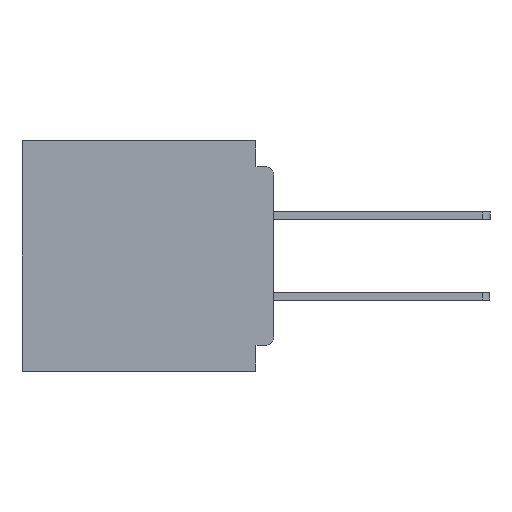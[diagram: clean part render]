
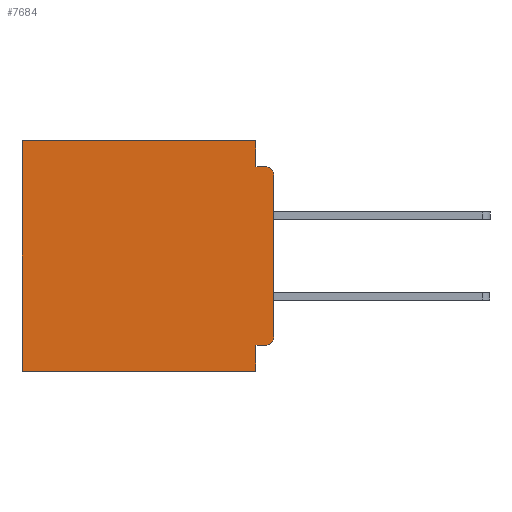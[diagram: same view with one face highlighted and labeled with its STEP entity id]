
A CAD part, left-side view. The second image highlights one B-rep face of the part: STEP entity #7684.
In plain terms, the highlighted planar face has unit normal (-1, 0, 0).
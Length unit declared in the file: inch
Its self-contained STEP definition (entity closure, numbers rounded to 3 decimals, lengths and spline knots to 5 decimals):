
#1303 = ORIENTED_EDGE ( 'NONE', *, *, #30740, .F. ) ;
#1503 = CARTESIAN_POINT ( 'NONE',  ( 0.3, 0.015, -0.045 ) ) ;
#1570 = CIRCLE ( 'NONE', #12042, 0.015 ) ;
#2046 = VECTOR ( 'NONE', #31930, 39.37008 ) ;
#2366 = VECTOR ( 'NONE', #34991, 39.37008 ) ;
#3516 = EDGE_CURVE ( 'NONE', #25555, #14391, #24596, .T. ) ;
#4709 = ORIENTED_EDGE ( 'NONE', *, *, #11764, .T. ) ;
#5438 = ORIENTED_EDGE ( 'NONE', *, *, #25407, .T. ) ;
#5734 = EDGE_CURVE ( 'NONE', #8645, #21257, #29737, .T. ) ;
#5780 = ORIENTED_EDGE ( 'NONE', *, *, #40398, .F. ) ;
#5955 = CARTESIAN_POINT ( 'NONE',  ( 0.3, 0.031, -0.4 ) ) ;
#6631 = EDGE_CURVE ( 'NONE', #18352, #15767, #32125, .T. ) ;
#7684 = ADVANCED_FACE ( 'NONE', ( #35059 ), #19772, .F. ) ;
#8597 = DIRECTION ( 'NONE',  ( 0., 1., 0. ) ) ;
#8645 = VERTEX_POINT ( 'NONE', #5955 ) ;
#8955 = VECTOR ( 'NONE', #8597, 39.37008 ) ;
#9021 = EDGE_CURVE ( 'NONE', #36735, #28432, #19978, .T. ) ;
#9938 = CARTESIAN_POINT ( 'NONE',  ( 0.3, 0.015, -0.06 ) ) ;
#11764 = EDGE_CURVE ( 'NONE', #18352, #17132, #48772, .T. ) ;
#12042 = AXIS2_PLACEMENT_3D ( 'NONE', #38717, #15432, #42617 ) ;
#12592 = VECTOR ( 'NONE', #44563, 39.37008 ) ;
#13933 = DIRECTION ( 'NONE',  ( 0., 0., -1. ) ) ;
#14184 = LINE ( 'NONE', #35160, #42783 ) ;
#14391 = VERTEX_POINT ( 'NONE', #43313 ) ;
#15432 = DIRECTION ( 'NONE',  ( -1., 0., 0. ) ) ;
#15767 = VERTEX_POINT ( 'NONE', #47376 ) ;
#16505 = DIRECTION ( 'NONE',  ( 0., -1., 0. ) ) ;
#16773 = LINE ( 'NONE', #39748, #37413 ) ;
#16956 = EDGE_CURVE ( 'NONE', #36735, #38547, #31691, .T. ) ;
#17132 = VERTEX_POINT ( 'NONE', #1503 ) ;
#18352 = VERTEX_POINT ( 'NONE', #43980 ) ;
#18750 = VECTOR ( 'NONE', #20859, 39.37008 ) ;
#19772 = PLANE ( 'NONE',  #39013 ) ;
#19978 = LINE ( 'NONE', #32343, #18750 ) ;
#20193 = VECTOR ( 'NONE', #35647, 39.37008 ) ;
#20577 = EDGE_LOOP ( 'NONE', ( #35927, #4709, #5780, #30472, #31351, #5438, #30314, #1303, #44318, #35629 ) ) ;
#20585 = CARTESIAN_POINT ( 'NONE',  ( 0.3, 0.437, 0. ) ) ;
#20859 = DIRECTION ( 'NONE',  ( 0., 0., -1. ) ) ;
#21257 = VERTEX_POINT ( 'NONE', #47696 ) ;
#21399 = CARTESIAN_POINT ( 'NONE',  ( 0.3, 0., -0.4 ) ) ;
#23464 = DIRECTION ( 'NONE',  ( 0., 0., -1. ) ) ;
#24596 = LINE ( 'NONE', #35058, #2366 ) ;
#25259 = AXIS2_PLACEMENT_3D ( 'NONE', #9938, #37262, #13933 ) ;
#25407 = EDGE_CURVE ( 'NONE', #38547, #21257, #33367, .T. ) ;
#25555 = VERTEX_POINT ( 'NONE', #32926 ) ;
#27368 = CARTESIAN_POINT ( 'NONE',  ( 0.3, 0., -0.4 ) ) ;
#27531 = DIRECTION ( 'NONE',  ( 0., 0., -1. ) ) ;
#28290 = CARTESIAN_POINT ( 'NONE',  ( 0.3, 0.031, 0. ) ) ;
#28432 = VERTEX_POINT ( 'NONE', #35299 ) ;
#29737 = LINE ( 'NONE', #47698, #8955 ) ;
#30314 = ORIENTED_EDGE ( 'NONE', *, *, #5734, .F. ) ;
#30472 = ORIENTED_EDGE ( 'NONE', *, *, #9021, .F. ) ;
#30740 = EDGE_CURVE ( 'NONE', #14391, #8645, #14184, .T. ) ;
#31351 = ORIENTED_EDGE ( 'NONE', *, *, #16956, .T. ) ;
#31691 = LINE ( 'NONE', #31722, #20193 ) ;
#31722 = CARTESIAN_POINT ( 'NONE',  ( 0.3, 0., 0. ) ) ;
#31930 = DIRECTION ( 'NONE',  ( 0., 0., -1. ) ) ;
#32125 = LINE ( 'NONE', #21399, #12592 ) ;
#32343 = CARTESIAN_POINT ( 'NONE',  ( 0.3, 0.031, 0. ) ) ;
#32926 = CARTESIAN_POINT ( 'NONE',  ( 0.3, 0.015, -0.355 ) ) ;
#33367 = LINE ( 'NONE', #39738, #2046 ) ;
#34991 = DIRECTION ( 'NONE',  ( 0., 1., 0. ) ) ;
#35058 = CARTESIAN_POINT ( 'NONE',  ( 0.3, 0., -0.355 ) ) ;
#35059 = FACE_OUTER_BOUND ( 'NONE', #20577, .T. ) ;
#35160 = CARTESIAN_POINT ( 'NONE',  ( 0.3, 0.031, -0.4 ) ) ;
#35299 = CARTESIAN_POINT ( 'NONE',  ( 0.3, 0.031, -0.045 ) ) ;
#35629 = ORIENTED_EDGE ( 'NONE', *, *, #43607, .T. ) ;
#35647 = DIRECTION ( 'NONE',  ( 0., 1., 0. ) ) ;
#35927 = ORIENTED_EDGE ( 'NONE', *, *, #6631, .F. ) ;
#36735 = VERTEX_POINT ( 'NONE', #28290 ) ;
#37262 = DIRECTION ( 'NONE',  ( -1., 0., 0. ) ) ;
#37413 = VECTOR ( 'NONE', #16505, 39.37008 ) ;
#38547 = VERTEX_POINT ( 'NONE', #20585 ) ;
#38717 = CARTESIAN_POINT ( 'NONE',  ( 0.3, 0.015, -0.34 ) ) ;
#39013 = AXIS2_PLACEMENT_3D ( 'NONE', #27368, #39093, #27531 ) ;
#39093 = DIRECTION ( 'NONE',  ( 1., 0., 0. ) ) ;
#39738 = CARTESIAN_POINT ( 'NONE',  ( 0.3, 0.437, -0.4 ) ) ;
#39748 = CARTESIAN_POINT ( 'NONE',  ( 0.3, 0., -0.045 ) ) ;
#40398 = EDGE_CURVE ( 'NONE', #28432, #17132, #16773, .T. ) ;
#42617 = DIRECTION ( 'NONE',  ( 0., 0., -1. ) ) ;
#42783 = VECTOR ( 'NONE', #23464, 39.37008 ) ;
#43313 = CARTESIAN_POINT ( 'NONE',  ( 0.3, 0.031, -0.355 ) ) ;
#43607 = EDGE_CURVE ( 'NONE', #25555, #15767, #1570, .T. ) ;
#43980 = CARTESIAN_POINT ( 'NONE',  ( 0.3, 0., -0.06 ) ) ;
#44318 = ORIENTED_EDGE ( 'NONE', *, *, #3516, .F. ) ;
#44563 = DIRECTION ( 'NONE',  ( 0., 0., -1. ) ) ;
#47376 = CARTESIAN_POINT ( 'NONE',  ( 0.3, 0., -0.34 ) ) ;
#47696 = CARTESIAN_POINT ( 'NONE',  ( 0.3, 0.437, -0.4 ) ) ;
#47698 = CARTESIAN_POINT ( 'NONE',  ( 0.3, 0., -0.4 ) ) ;
#48772 = CIRCLE ( 'NONE', #25259, 0.015 ) ;
